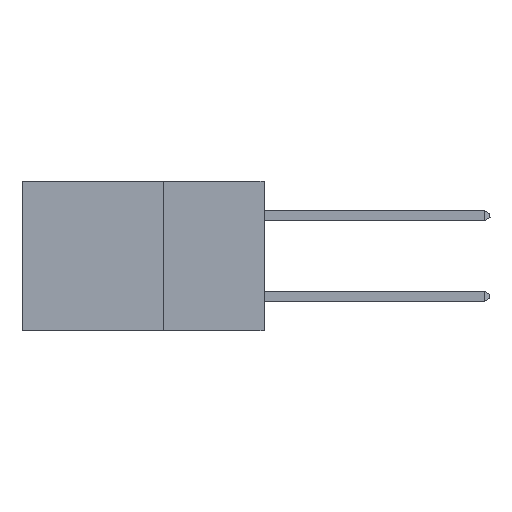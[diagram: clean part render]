
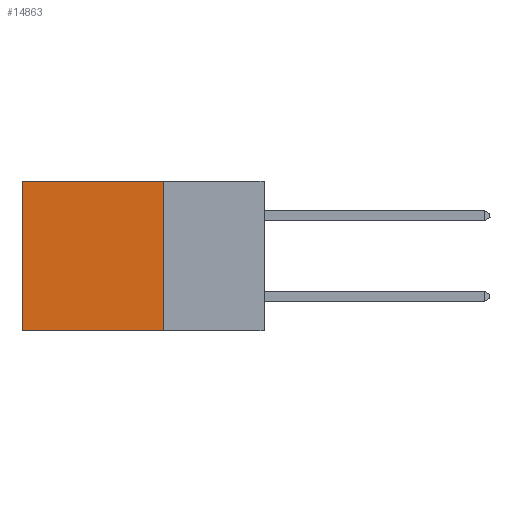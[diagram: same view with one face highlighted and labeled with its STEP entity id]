
A CAD part, left-side view. The second image highlights one B-rep face of the part: STEP entity #14863.
In plain terms, the highlighted planar face has unit normal (-1, 0, 0).
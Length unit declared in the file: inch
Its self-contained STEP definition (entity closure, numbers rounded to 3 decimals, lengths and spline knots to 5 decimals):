
#397 = CARTESIAN_POINT ( 'NONE',  ( 0.298, 0.25, 0. ) ) ;
#1455 = EDGE_CURVE ( 'NONE', #6987, #3821, #3075, .T. ) ;
#2310 = CARTESIAN_POINT ( 'NONE',  ( 0.298, 0.25, -0.37 ) ) ;
#2474 = FACE_OUTER_BOUND ( 'NONE', #10396, .T. ) ;
#2812 = CARTESIAN_POINT ( 'NONE',  ( 0.298, 0.25, 0. ) ) ;
#2973 = EDGE_CURVE ( 'NONE', #15689, #12678, #8949, .T. ) ;
#3075 = LINE ( 'NONE', #11897, #13620 ) ;
#3797 = VECTOR ( 'NONE', #9795, 39.37008 ) ;
#3821 = VERTEX_POINT ( 'NONE', #15337 ) ;
#4153 = EDGE_CURVE ( 'NONE', #15689, #6987, #13741, .T. ) ;
#4178 = CARTESIAN_POINT ( 'NONE',  ( 0.298, 0.6, 0. ) ) ;
#5896 = ORIENTED_EDGE ( 'NONE', *, *, #6355, .F. ) ;
#6260 = VECTOR ( 'NONE', #17458, 39.37008 ) ;
#6355 = EDGE_CURVE ( 'NONE', #12678, #3821, #7556, .T. ) ;
#6987 = VERTEX_POINT ( 'NONE', #4178 ) ;
#7556 = LINE ( 'NONE', #2310, #3797 ) ;
#7855 = AXIS2_PLACEMENT_3D ( 'NONE', #13928, #18175, #8456 ) ;
#8456 = DIRECTION ( 'NONE',  ( 0., 0., -1. ) ) ;
#8949 = LINE ( 'NONE', #2812, #9402 ) ;
#9388 = ORIENTED_EDGE ( 'NONE', *, *, #1455, .T. ) ;
#9402 = VECTOR ( 'NONE', #11422, 39.37008 ) ;
#9795 = DIRECTION ( 'NONE',  ( 0., 1., 0. ) ) ;
#10295 = DIRECTION ( 'NONE',  ( 0., 0., -1. ) ) ;
#10396 = EDGE_LOOP ( 'NONE', ( #9388, #5896, #11557, #11067 ) ) ;
#11067 = ORIENTED_EDGE ( 'NONE', *, *, #4153, .T. ) ;
#11205 = PLANE ( 'NONE',  #7855 ) ;
#11422 = DIRECTION ( 'NONE',  ( 0., 0., -1. ) ) ;
#11557 = ORIENTED_EDGE ( 'NONE', *, *, #2973, .F. ) ;
#11897 = CARTESIAN_POINT ( 'NONE',  ( 0.298, 0.6, 0. ) ) ;
#12675 = CARTESIAN_POINT ( 'NONE',  ( 0.298, 0.25, -0.37 ) ) ;
#12678 = VERTEX_POINT ( 'NONE', #12675 ) ;
#13620 = VECTOR ( 'NONE', #10295, 39.37008 ) ;
#13741 = LINE ( 'NONE', #397, #6260 ) ;
#13928 = CARTESIAN_POINT ( 'NONE',  ( 0.298, 0.25, 0. ) ) ;
#14863 = ADVANCED_FACE ( 'NONE', ( #2474 ), #11205, .F. ) ;
#15337 = CARTESIAN_POINT ( 'NONE',  ( 0.298, 0.6, -0.37 ) ) ;
#15552 = CARTESIAN_POINT ( 'NONE',  ( 0.298, 0.25, 0. ) ) ;
#15689 = VERTEX_POINT ( 'NONE', #15552 ) ;
#17458 = DIRECTION ( 'NONE',  ( 0., 1., 0. ) ) ;
#18175 = DIRECTION ( 'NONE',  ( 1., 0., 0. ) ) ;
